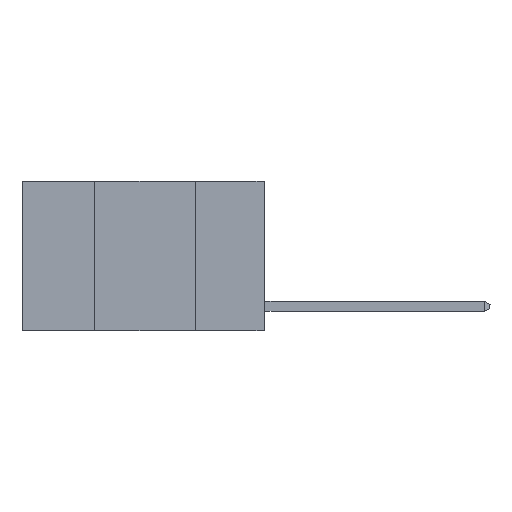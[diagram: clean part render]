
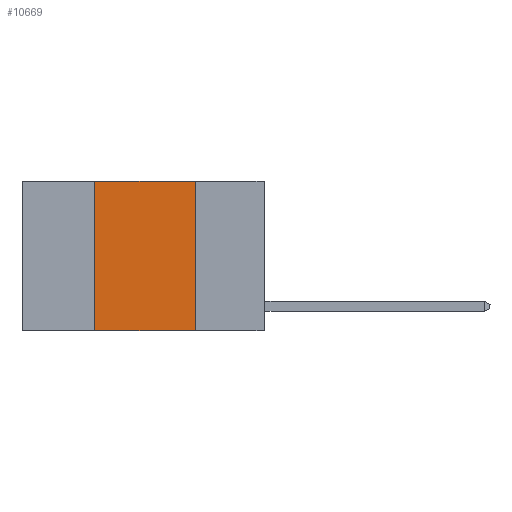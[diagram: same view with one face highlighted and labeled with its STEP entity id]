
A CAD part, left-side view. The second image highlights one B-rep face of the part: STEP entity #10669.
In plain terms, the highlighted planar face has unit normal (-1, 0, 0).
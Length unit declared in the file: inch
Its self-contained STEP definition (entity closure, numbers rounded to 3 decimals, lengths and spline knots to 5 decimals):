
#220 = EDGE_LOOP ( 'NONE', ( #18731, #21364, #4808, #13824 ) ) ;
#2366 = PLANE ( 'NONE',  #8217 ) ;
#3885 = DIRECTION ( 'NONE',  ( 0., 0., 1. ) ) ;
#4575 = CARTESIAN_POINT ( 'NONE',  ( 0., 0.6, 0. ) ) ;
#4808 = ORIENTED_EDGE ( 'NONE', *, *, #28078, .F. ) ;
#4838 = LINE ( 'NONE', #7329, #22480 ) ;
#6044 = CARTESIAN_POINT ( 'NONE',  ( 0., 0.42, 0. ) ) ;
#6570 = EDGE_CURVE ( 'NONE', #13134, #21968, #4838, .T. ) ;
#6820 = DIRECTION ( 'NONE',  ( 1., 0., 0. ) ) ;
#7329 = CARTESIAN_POINT ( 'NONE',  ( 0., 0.6, 0. ) ) ;
#8217 = AXIS2_PLACEMENT_3D ( 'NONE', #4575, #6820, #21740 ) ;
#8425 = CARTESIAN_POINT ( 'NONE',  ( 0., 0.17, 0. ) ) ;
#9488 = EDGE_CURVE ( 'NONE', #20382, #21651, #16374, .T. ) ;
#10335 = CARTESIAN_POINT ( 'NONE',  ( 0., 0.42, -0.37 ) ) ;
#10669 = ADVANCED_FACE ( 'NONE', ( #13556 ), #2366, .F. ) ;
#11393 = CARTESIAN_POINT ( 'NONE',  ( 0., 0.17, 0. ) ) ;
#11678 = VECTOR ( 'NONE', #19532, 39.37008 ) ;
#11715 = CARTESIAN_POINT ( 'NONE',  ( 0., 0.17, -0.37 ) ) ;
#12907 = VECTOR ( 'NONE', #3885, 39.37008 ) ;
#13134 = VERTEX_POINT ( 'NONE', #6044 ) ;
#13556 = FACE_OUTER_BOUND ( 'NONE', #220, .T. ) ;
#13824 = ORIENTED_EDGE ( 'NONE', *, *, #9488, .T. ) ;
#16374 = LINE ( 'NONE', #23411, #26429 ) ;
#18731 = ORIENTED_EDGE ( 'NONE', *, *, #24719, .F. ) ;
#19155 = CARTESIAN_POINT ( 'NONE',  ( 0., 0.42, 0. ) ) ;
#19532 = DIRECTION ( 'NONE',  ( 0., 0., -1. ) ) ;
#20382 = VERTEX_POINT ( 'NONE', #10335 ) ;
#21364 = ORIENTED_EDGE ( 'NONE', *, *, #6570, .F. ) ;
#21379 = DIRECTION ( 'NONE',  ( 0., -1., 0. ) ) ;
#21651 = VERTEX_POINT ( 'NONE', #11715 ) ;
#21740 = DIRECTION ( 'NONE',  ( 0., 0., -1. ) ) ;
#21968 = VERTEX_POINT ( 'NONE', #8425 ) ;
#22480 = VECTOR ( 'NONE', #27153, 39.37008 ) ;
#22764 = LINE ( 'NONE', #11393, #11678 ) ;
#23411 = CARTESIAN_POINT ( 'NONE',  ( 0., 0.6, -0.37 ) ) ;
#24323 = LINE ( 'NONE', #19155, #12907 ) ;
#24719 = EDGE_CURVE ( 'NONE', #21968, #21651, #22764, .T. ) ;
#26429 = VECTOR ( 'NONE', #21379, 39.37008 ) ;
#27153 = DIRECTION ( 'NONE',  ( 0., -1., 0. ) ) ;
#28078 = EDGE_CURVE ( 'NONE', #20382, #13134, #24323, .T. ) ;
